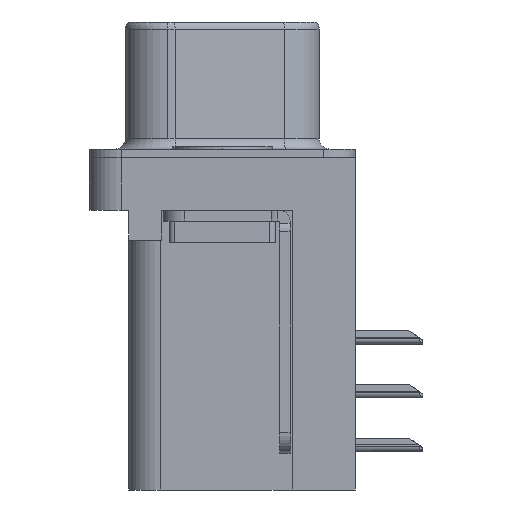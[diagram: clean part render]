
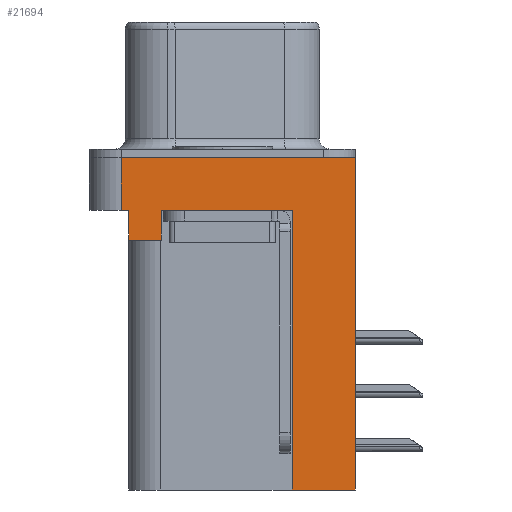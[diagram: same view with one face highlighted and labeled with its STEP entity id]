
A CAD part, left-side view. The second image highlights one B-rep face of the part: STEP entity #21694.
In plain terms, the highlighted planar face has unit normal (-1, 0, 0).
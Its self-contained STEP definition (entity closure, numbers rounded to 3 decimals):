
#449 = ORIENTED_EDGE ( 'NONE', *, *, #23037, .F. ) ;
#869 = LINE ( 'NONE', #10085, #6671 ) ;
#1780 = VERTEX_POINT ( 'NONE', #18269 ) ;
#2345 = VERTEX_POINT ( 'NONE', #8887 ) ;
#2835 = VECTOR ( 'NONE', #15252, 1000. ) ;
#2871 = DIRECTION ( 'NONE',  ( 0., -1., 0. ) ) ;
#3628 = LINE ( 'NONE', #19757, #29807 ) ;
#3757 = LINE ( 'NONE', #20861, #16146 ) ;
#4279 = CARTESIAN_POINT ( 'NONE',  ( -2.91, -6.275, -2.5 ) ) ;
#4330 = VERTEX_POINT ( 'NONE', #12580 ) ;
#4387 = DIRECTION ( 'NONE',  ( 0., 0., 1. ) ) ;
#4450 = CARTESIAN_POINT ( 'NONE',  ( -2.91, -3.295, -15.7 ) ) ;
#5834 = DIRECTION ( 'NONE',  ( 0., 0., 1. ) ) ;
#6671 = VECTOR ( 'NONE', #25504, 1000. ) ;
#6787 = FACE_OUTER_BOUND ( 'NONE', #24088, .T. ) ;
#7641 = ORIENTED_EDGE ( 'NONE', *, *, #26431, .F. ) ;
#8887 = CARTESIAN_POINT ( 'NONE',  ( -2.91, 4.775, 0. ) ) ;
#10085 = CARTESIAN_POINT ( 'NONE',  ( -2.91, 4.425, -3.9 ) ) ;
#10192 = AXIS2_PLACEMENT_3D ( 'NONE', #11495, #29419, #14002 ) ;
#10196 = LINE ( 'NONE', #12822, #2835 ) ;
#10460 = CARTESIAN_POINT ( 'NONE',  ( -2.91, 4.425, -2.5 ) ) ;
#11056 = VECTOR ( 'NONE', #28565, 1000. ) ;
#11209 = CARTESIAN_POINT ( 'NONE',  ( -2.91, -6.275, -2.5 ) ) ;
#11495 = CARTESIAN_POINT ( 'NONE',  ( -2.91, -6.275, -2.5 ) ) ;
#11598 = ORIENTED_EDGE ( 'NONE', *, *, #23349, .F. ) ;
#11819 = LINE ( 'NONE', #23187, #11056 ) ;
#12260 = DIRECTION ( 'NONE',  ( 0., -1., 0. ) ) ;
#12580 = CARTESIAN_POINT ( 'NONE',  ( -2.91, -3.295, -2.5 ) ) ;
#12822 = CARTESIAN_POINT ( 'NONE',  ( -2.91, 4.425, -3.9 ) ) ;
#13534 = ORIENTED_EDGE ( 'NONE', *, *, #22852, .T. ) ;
#13897 = PLANE ( 'NONE',  #10192 ) ;
#13903 = ORIENTED_EDGE ( 'NONE', *, *, #28601, .F. ) ;
#14002 = DIRECTION ( 'NONE',  ( 0., 0., 1. ) ) ;
#14822 = VECTOR ( 'NONE', #32134, 1000. ) ;
#14874 = VERTEX_POINT ( 'NONE', #32362 ) ;
#15064 = ORIENTED_EDGE ( 'NONE', *, *, #22989, .T. ) ;
#15252 = DIRECTION ( 'NONE',  ( 0., 0., 1. ) ) ;
#15253 = VERTEX_POINT ( 'NONE', #25979 ) ;
#16146 = VECTOR ( 'NONE', #5834, 1000. ) ;
#16735 = CARTESIAN_POINT ( 'NONE',  ( -2.91, 2.895, -3.9 ) ) ;
#17137 = VECTOR ( 'NONE', #21346, 1000. ) ;
#17689 = CARTESIAN_POINT ( 'NONE',  ( -2.91, -6.275, 0. ) ) ;
#17896 = VERTEX_POINT ( 'NONE', #25081 ) ;
#17920 = LINE ( 'NONE', #11209, #17137 ) ;
#18269 = CARTESIAN_POINT ( 'NONE',  ( -2.91, 4.425, -3.9 ) ) ;
#18576 = ORIENTED_EDGE ( 'NONE', *, *, #22886, .F. ) ;
#19757 = CARTESIAN_POINT ( 'NONE',  ( -2.91, -6.275, -2.5 ) ) ;
#19804 = VECTOR ( 'NONE', #4387, 1000. ) ;
#19967 = VERTEX_POINT ( 'NONE', #4450 ) ;
#20365 = VECTOR ( 'NONE', #2871, 1000. ) ;
#20630 = VECTOR ( 'NONE', #29563, 1000. ) ;
#20861 = CARTESIAN_POINT ( 'NONE',  ( -2.91, -3.295, -15.7 ) ) ;
#20993 = CARTESIAN_POINT ( 'NONE',  ( -2.91, -6.275, -15.7 ) ) ;
#21346 = DIRECTION ( 'NONE',  ( 0., -1., 0. ) ) ;
#21500 = VERTEX_POINT ( 'NONE', #20993 ) ;
#21556 = CARTESIAN_POINT ( 'NONE',  ( -2.91, 4.775, -2.5 ) ) ;
#21568 = LINE ( 'NONE', #21556, #14822 ) ;
#21694 = ADVANCED_FACE ( 'NONE', ( #6787 ), #13897, .T. ) ;
#22852 = EDGE_CURVE ( 'NONE', #24927, #25783, #3628, .T. ) ;
#22886 = EDGE_CURVE ( 'NONE', #1780, #25783, #10196, .T. ) ;
#22989 = EDGE_CURVE ( 'NONE', #17896, #4330, #17920, .T. ) ;
#23037 = EDGE_CURVE ( 'NONE', #24927, #2345, #21568, .T. ) ;
#23187 = CARTESIAN_POINT ( 'NONE',  ( -2.91, -3.295, -15.7 ) ) ;
#23349 = EDGE_CURVE ( 'NONE', #2345, #15253, #26448, .T. ) ;
#24088 = EDGE_LOOP ( 'NONE', ( #11598, #449, #13534, #18576, #13903, #25904, #15064, #7641, #26971, #25141 ) ) ;
#24586 = EDGE_CURVE ( 'NONE', #21500, #15253, #28357, .T. ) ;
#24602 = EDGE_CURVE ( 'NONE', #14874, #17896, #27508, .T. ) ;
#24927 = VERTEX_POINT ( 'NONE', #28501 ) ;
#25081 = CARTESIAN_POINT ( 'NONE',  ( -2.91, 2.895, -2.5 ) ) ;
#25141 = ORIENTED_EDGE ( 'NONE', *, *, #24586, .T. ) ;
#25504 = DIRECTION ( 'NONE',  ( 0., 1., 0. ) ) ;
#25783 = VERTEX_POINT ( 'NONE', #10460 ) ;
#25904 = ORIENTED_EDGE ( 'NONE', *, *, #24602, .T. ) ;
#25979 = CARTESIAN_POINT ( 'NONE',  ( -2.91, -6.275, 0. ) ) ;
#26431 = EDGE_CURVE ( 'NONE', #19967, #4330, #3757, .T. ) ;
#26448 = LINE ( 'NONE', #17689, #20365 ) ;
#26873 = EDGE_CURVE ( 'NONE', #21500, #19967, #11819, .T. ) ;
#26971 = ORIENTED_EDGE ( 'NONE', *, *, #26873, .F. ) ;
#27508 = LINE ( 'NONE', #16735, #19804 ) ;
#28357 = LINE ( 'NONE', #4279, #20630 ) ;
#28501 = CARTESIAN_POINT ( 'NONE',  ( -2.91, 4.775, -2.5 ) ) ;
#28565 = DIRECTION ( 'NONE',  ( 0., 1., 0. ) ) ;
#28601 = EDGE_CURVE ( 'NONE', #14874, #1780, #869, .T. ) ;
#29419 = DIRECTION ( 'NONE',  ( -1., 0., 0. ) ) ;
#29563 = DIRECTION ( 'NONE',  ( 0., 0., 1. ) ) ;
#29807 = VECTOR ( 'NONE', #12260, 1000. ) ;
#32134 = DIRECTION ( 'NONE',  ( 0., 0., 1. ) ) ;
#32362 = CARTESIAN_POINT ( 'NONE',  ( -2.91, 2.895, -3.9 ) ) ;
